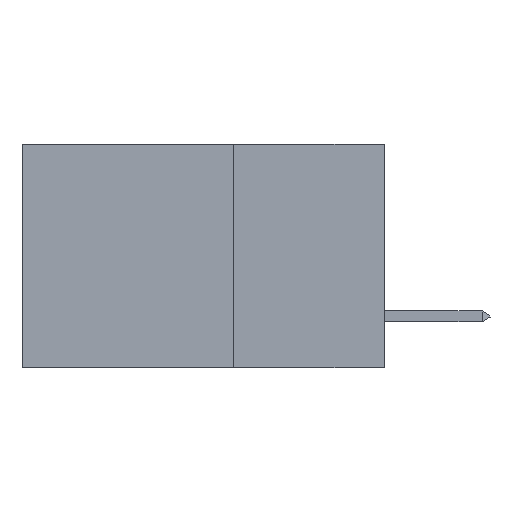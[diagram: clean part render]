
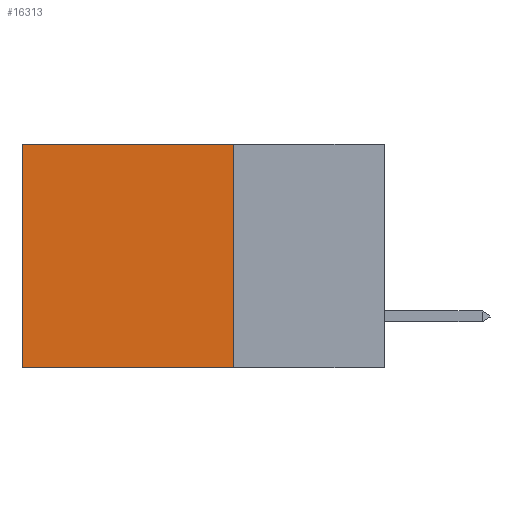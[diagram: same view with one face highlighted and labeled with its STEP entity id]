
A CAD part, left-side view. The second image highlights one B-rep face of the part: STEP entity #16313.
In plain terms, the highlighted planar face has unit normal (-1, 0, 0).
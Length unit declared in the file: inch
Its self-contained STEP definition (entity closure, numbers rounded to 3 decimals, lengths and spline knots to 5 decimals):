
#1731 = AXIS2_PLACEMENT_3D ( 'NONE', #16329, #3944, #20569 ) ;
#3944 = DIRECTION ( 'NONE',  ( 1., 0., 0. ) ) ;
#4683 = CARTESIAN_POINT ( 'NONE',  ( 0.2875, 0.6, -0.37 ) ) ;
#6334 = CARTESIAN_POINT ( 'NONE',  ( 0.2875, 0.25, 0. ) ) ;
#7485 = VERTEX_POINT ( 'NONE', #6334 ) ;
#8031 = ORIENTED_EDGE ( 'NONE', *, *, #12839, .T. ) ;
#8637 = EDGE_CURVE ( 'NONE', #7485, #10134, #19270, .T. ) ;
#8866 = EDGE_CURVE ( 'NONE', #10134, #10087, #17646, .T. ) ;
#9144 = DIRECTION ( 'NONE',  ( 0., 0., -1. ) ) ;
#9667 = DIRECTION ( 'NONE',  ( 0., 0., -1. ) ) ;
#10087 = VERTEX_POINT ( 'NONE', #4683 ) ;
#10134 = VERTEX_POINT ( 'NONE', #21041 ) ;
#10441 = DIRECTION ( 'NONE',  ( 0., 1., 0. ) ) ;
#10907 = CARTESIAN_POINT ( 'NONE',  ( 0.2875, 0.25, -0.37 ) ) ;
#11476 = FACE_OUTER_BOUND ( 'NONE', #17691, .T. ) ;
#12511 = PLANE ( 'NONE',  #1731 ) ;
#12839 = EDGE_CURVE ( 'NONE', #26171, #10087, #22280, .T. ) ;
#14185 = VECTOR ( 'NONE', #9144, 39.37008 ) ;
#14216 = ORIENTED_EDGE ( 'NONE', *, *, #8866, .F. ) ;
#15073 = VECTOR ( 'NONE', #9667, 39.37008 ) ;
#15702 = VECTOR ( 'NONE', #19052, 39.37008 ) ;
#16313 = ADVANCED_FACE ( 'NONE', ( #11476 ), #12511, .F. ) ;
#16329 = CARTESIAN_POINT ( 'NONE',  ( 0.2875, 0.25, 0. ) ) ;
#16591 = CARTESIAN_POINT ( 'NONE',  ( 0.2875, 0.25, 0. ) ) ;
#17493 = ORIENTED_EDGE ( 'NONE', *, *, #22992, .T. ) ;
#17646 = LINE ( 'NONE', #10907, #15702 ) ;
#17691 = EDGE_LOOP ( 'NONE', ( #8031, #14216, #20711, #17493 ) ) ;
#19052 = DIRECTION ( 'NONE',  ( 0., 1., 0. ) ) ;
#19217 = CARTESIAN_POINT ( 'NONE',  ( 0.2875, 0.6, 0. ) ) ;
#19267 = VECTOR ( 'NONE', #10441, 39.37008 ) ;
#19270 = LINE ( 'NONE', #24214, #15073 ) ;
#20569 = DIRECTION ( 'NONE',  ( 0., 0., -1. ) ) ;
#20711 = ORIENTED_EDGE ( 'NONE', *, *, #8637, .F. ) ;
#21041 = CARTESIAN_POINT ( 'NONE',  ( 0.2875, 0.25, -0.37 ) ) ;
#21871 = LINE ( 'NONE', #16591, #19267 ) ;
#22280 = LINE ( 'NONE', #23773, #14185 ) ;
#22992 = EDGE_CURVE ( 'NONE', #7485, #26171, #21871, .T. ) ;
#23773 = CARTESIAN_POINT ( 'NONE',  ( 0.2875, 0.6, 0. ) ) ;
#24214 = CARTESIAN_POINT ( 'NONE',  ( 0.2875, 0.25, 0. ) ) ;
#26171 = VERTEX_POINT ( 'NONE', #19217 ) ;
